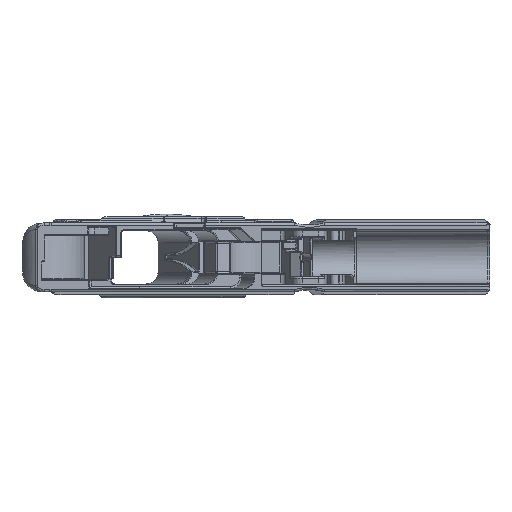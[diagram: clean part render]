
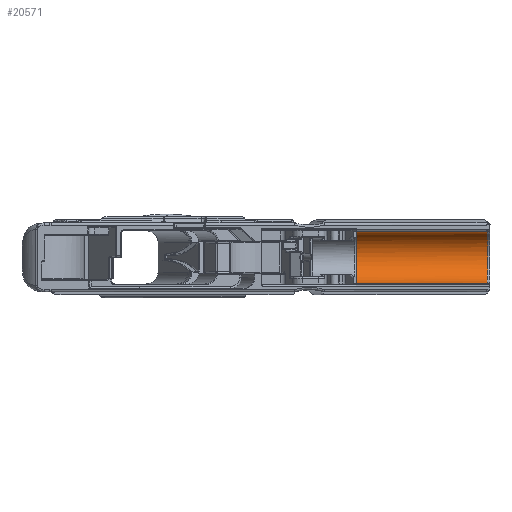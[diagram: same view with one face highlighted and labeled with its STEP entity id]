
A CAD part, front view. The second image highlights one B-rep face of the part: STEP entity #20571.
In plain terms, the highlighted cylindrical face has radius 8.75 mm (diameter 17.5 mm), a partial arc.
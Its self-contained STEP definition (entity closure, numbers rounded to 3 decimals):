
#600=B_SPLINE_CURVE_WITH_KNOTS('',3,(#33116,#33117,#33118,#33119),
 .UNSPECIFIED.,.F.,.F.,(4,4),(0.,1.),.UNSPECIFIED.);
#601=B_SPLINE_CURVE_WITH_KNOTS('',3,(#33127,#33128,#33129,#33130),
 .UNSPECIFIED.,.F.,.F.,(4,4),(0.,1.),.UNSPECIFIED.);
#2176=FACE_OUTER_BOUND('',#3488,.T.);
#3488=EDGE_LOOP('',(#13824,#13825,#13826,#13827,#13828,#13829,#13830,#13831));
#4853=CIRCLE('',#22040,8.75);
#5538=LINE('',#33114,#6643);
#5539=LINE('',#33121,#6644);
#5540=LINE('',#33125,#6645);
#5541=LINE('',#33131,#6646);
#6643=VECTOR('',#24211,1000.);
#6644=VECTOR('',#24212,1000.);
#6645=VECTOR('',#24215,1000.);
#6646=VECTOR('',#24216,1000.);
#7699=ELLIPSE('',#22039,8.751,8.75);
#8329=VERTEX_POINT('',#33110);
#8330=VERTEX_POINT('',#33111);
#8331=VERTEX_POINT('',#33113);
#8332=VERTEX_POINT('',#33115);
#8333=VERTEX_POINT('',#33120);
#8334=VERTEX_POINT('',#33122);
#8335=VERTEX_POINT('',#33124);
#8336=VERTEX_POINT('',#33126);
#10399=EDGE_CURVE('',#8329,#8330,#7699,.T.);
#10400=EDGE_CURVE('',#8329,#8331,#5538,.T.);
#10401=EDGE_CURVE('',#8331,#8332,#600,.T.);
#10402=EDGE_CURVE('',#8332,#8333,#5539,.T.);
#10403=EDGE_CURVE('',#8334,#8333,#4853,.T.);
#10404=EDGE_CURVE('',#8335,#8334,#5540,.T.);
#10405=EDGE_CURVE('',#8335,#8336,#601,.T.);
#10406=EDGE_CURVE('',#8336,#8330,#5541,.T.);
#13824=ORIENTED_EDGE('',*,*,#10399,.F.);
#13825=ORIENTED_EDGE('',*,*,#10400,.T.);
#13826=ORIENTED_EDGE('',*,*,#10401,.T.);
#13827=ORIENTED_EDGE('',*,*,#10402,.T.);
#13828=ORIENTED_EDGE('',*,*,#10403,.F.);
#13829=ORIENTED_EDGE('',*,*,#10404,.F.);
#13830=ORIENTED_EDGE('',*,*,#10405,.T.);
#13831=ORIENTED_EDGE('',*,*,#10406,.T.);
#20098=CYLINDRICAL_SURFACE('',#22038,8.75);
#20571=ADVANCED_FACE('',(#2176),#20098,.F.);
#22038=AXIS2_PLACEMENT_3D('',#33109,#24207,#24208);
#22039=AXIS2_PLACEMENT_3D('',#33112,#24209,#24210);
#22040=AXIS2_PLACEMENT_3D('',#33123,#24213,#24214);
#24207=DIRECTION('center_axis',(-1.,0.,0.));
#24208=DIRECTION('ref_axis',(0.,1.,0.));
#24209=DIRECTION('center_axis',(-1.,0.017,0.));
#24210=DIRECTION('ref_axis',(0.017,1.,0.));
#24211=DIRECTION('',(-1.,0.,0.));
#24212=DIRECTION('',(1.,0.,0.));
#24213=DIRECTION('center_axis',(1.,0.,0.));
#24214=DIRECTION('ref_axis',(0.,1.,0.));
#24215=DIRECTION('',(1.,0.,0.));
#24216=DIRECTION('',(1.,0.,0.));
#33109=CARTESIAN_POINT('Origin',(157.53,5.96,0.));
#33110=CARTESIAN_POINT('',(156.586,5.96,8.75));
#33111=CARTESIAN_POINT('',(156.586,5.96,-8.75));
#33112=CARTESIAN_POINT('Origin',(156.586,5.96,0.));
#33113=CARTESIAN_POINT('',(112.522,5.96,8.75));
#33114=CARTESIAN_POINT('',(157.53,5.96,8.75));
#33115=CARTESIAN_POINT('',(112.522,6.21,8.748));
#33116=CARTESIAN_POINT('Ctrl Pts',(112.522,5.96,8.75));
#33117=CARTESIAN_POINT('Ctrl Pts',(112.522,6.043,8.75));
#33118=CARTESIAN_POINT('Ctrl Pts',(112.522,6.127,8.749));
#33119=CARTESIAN_POINT('Ctrl Pts',(112.522,6.21,8.748));
#33120=CARTESIAN_POINT('',(112.999,6.21,8.746));
#33121=CARTESIAN_POINT('',(112.999,6.21,8.746));
#33122=CARTESIAN_POINT('',(112.999,6.21,-8.746));
#33123=CARTESIAN_POINT('Origin',(112.999,5.96,0.));
#33124=CARTESIAN_POINT('',(112.522,6.21,-8.748));
#33125=CARTESIAN_POINT('',(157.53,6.21,-8.746));
#33126=CARTESIAN_POINT('',(112.522,5.96,-8.75));
#33127=CARTESIAN_POINT('Ctrl Pts',(112.522,6.21,-8.748));
#33128=CARTESIAN_POINT('Ctrl Pts',(112.522,6.127,-8.749));
#33129=CARTESIAN_POINT('Ctrl Pts',(112.522,6.043,-8.75));
#33130=CARTESIAN_POINT('Ctrl Pts',(112.522,5.96,-8.75));
#33131=CARTESIAN_POINT('',(157.53,5.96,-8.75));
